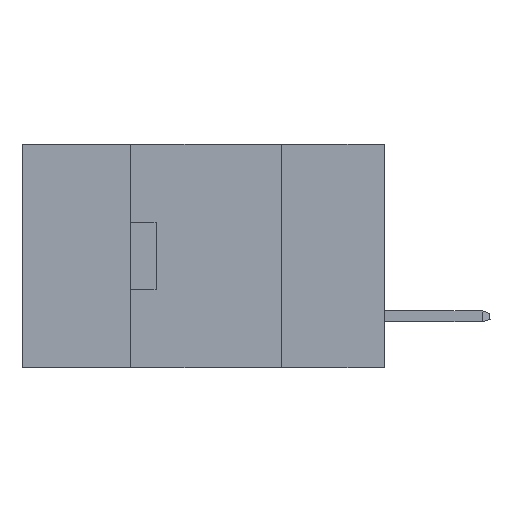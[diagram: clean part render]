
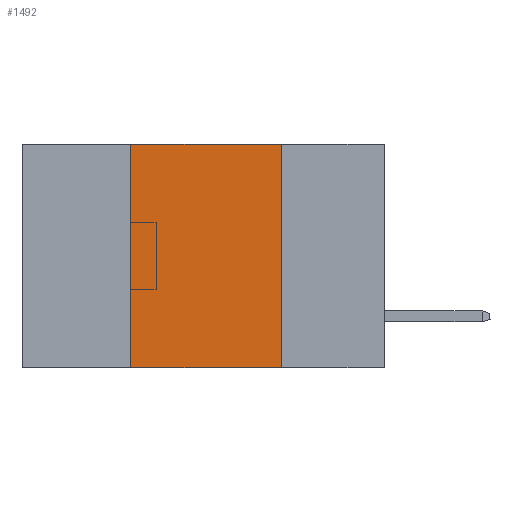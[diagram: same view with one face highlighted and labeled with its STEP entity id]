
A CAD part, left-side view. The second image highlights one B-rep face of the part: STEP entity #1492.
In plain terms, the highlighted planar face has unit normal (-1, 0, 0).
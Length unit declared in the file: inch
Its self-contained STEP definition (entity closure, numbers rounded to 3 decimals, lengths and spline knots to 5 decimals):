
#1196 = EDGE_CURVE ( 'NONE', #22734, #18153, #4833, .T. ) ;
#1492 = ADVANCED_FACE ( 'NONE', ( #3179 ), #15448, .F. ) ;
#3179 = FACE_OUTER_BOUND ( 'NONE', #5666, .T. ) ;
#3329 = CARTESIAN_POINT ( 'NONE',  ( 0., 0.42, 0. ) ) ;
#4833 = LINE ( 'NONE', #21594, #15911 ) ;
#5022 = CARTESIAN_POINT ( 'NONE',  ( 0., 0.6, -0.37 ) ) ;
#5066 = LINE ( 'NONE', #17780, #9990 ) ;
#5666 = EDGE_LOOP ( 'NONE', ( #8714, #15572, #12674, #13324 ) ) ;
#6345 = VERTEX_POINT ( 'NONE', #14005 ) ;
#7062 = LINE ( 'NONE', #23383, #12643 ) ;
#8034 = AXIS2_PLACEMENT_3D ( 'NONE', #15669, #15322, #15083 ) ;
#8714 = ORIENTED_EDGE ( 'NONE', *, *, #10343, .F. ) ;
#8960 = DIRECTION ( 'NONE',  ( 0., -1., 0. ) ) ;
#9990 = VECTOR ( 'NONE', #21771, 39.37008 ) ;
#10343 = EDGE_CURVE ( 'NONE', #6345, #17540, #5066, .T. ) ;
#11336 = DIRECTION ( 'NONE',  ( 0., -1., 0. ) ) ;
#11550 = EDGE_CURVE ( 'NONE', #22734, #17540, #11857, .T. ) ;
#11857 = LINE ( 'NONE', #5022, #22703 ) ;
#12643 = VECTOR ( 'NONE', #8960, 39.37008 ) ;
#12674 = ORIENTED_EDGE ( 'NONE', *, *, #1196, .F. ) ;
#13324 = ORIENTED_EDGE ( 'NONE', *, *, #11550, .T. ) ;
#14005 = CARTESIAN_POINT ( 'NONE',  ( 0., 0.17, 0. ) ) ;
#15083 = DIRECTION ( 'NONE',  ( 0., 0., -1. ) ) ;
#15322 = DIRECTION ( 'NONE',  ( 1., 0., 0. ) ) ;
#15448 = PLANE ( 'NONE',  #8034 ) ;
#15572 = ORIENTED_EDGE ( 'NONE', *, *, #20484, .F. ) ;
#15669 = CARTESIAN_POINT ( 'NONE',  ( 0., 0.6, 0. ) ) ;
#15911 = VECTOR ( 'NONE', #21754, 39.37008 ) ;
#17540 = VERTEX_POINT ( 'NONE', #23710 ) ;
#17780 = CARTESIAN_POINT ( 'NONE',  ( 0., 0.17, -0.37 ) ) ;
#18153 = VERTEX_POINT ( 'NONE', #3329 ) ;
#20484 = EDGE_CURVE ( 'NONE', #18153, #6345, #7062, .T. ) ;
#21594 = CARTESIAN_POINT ( 'NONE',  ( 0., 0.42, -0.37 ) ) ;
#21754 = DIRECTION ( 'NONE',  ( 0., 0., 1. ) ) ;
#21771 = DIRECTION ( 'NONE',  ( 0., 0., -1. ) ) ;
#22703 = VECTOR ( 'NONE', #11336, 39.37008 ) ;
#22734 = VERTEX_POINT ( 'NONE', #26504 ) ;
#23383 = CARTESIAN_POINT ( 'NONE',  ( 0., 0.6, 0. ) ) ;
#23710 = CARTESIAN_POINT ( 'NONE',  ( 0., 0.17, -0.37 ) ) ;
#26504 = CARTESIAN_POINT ( 'NONE',  ( 0., 0.42, -0.37 ) ) ;
